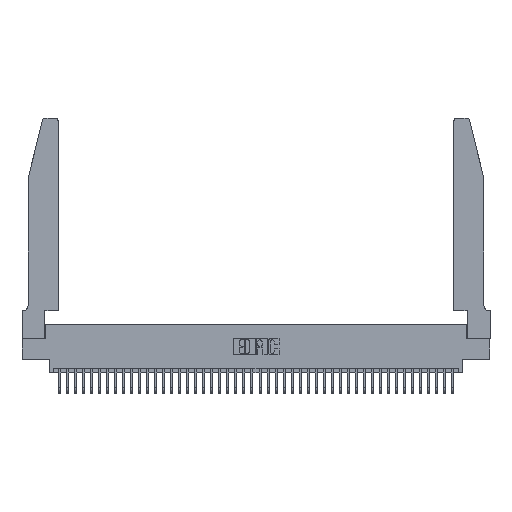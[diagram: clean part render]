
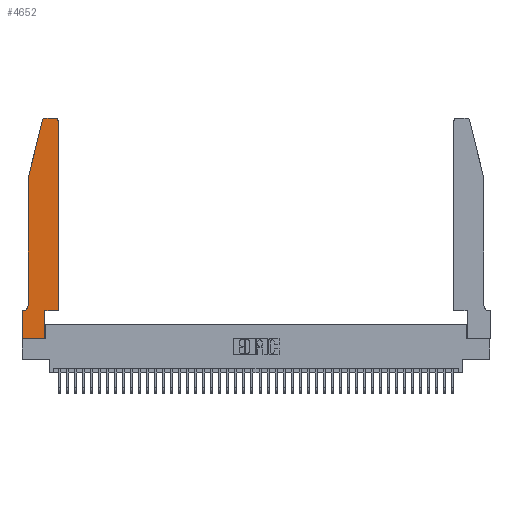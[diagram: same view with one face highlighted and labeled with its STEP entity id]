
A CAD part, top view. The second image highlights one B-rep face of the part: STEP entity #4652.
In plain terms, the highlighted planar face has unit normal (0, 0, 1).
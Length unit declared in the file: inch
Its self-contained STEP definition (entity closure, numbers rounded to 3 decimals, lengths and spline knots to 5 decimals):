
#1 = ORIENTED_EDGE ( 'NONE', *, *, #5140, .T. ) ;
#418 = CARTESIAN_POINT ( 'NONE',  ( 0.0755, 2., 0.37 ) ) ;
#725 = DIRECTION ( 'NONE',  ( -1., 0., 0. ) ) ;
#777 = EDGE_CURVE ( 'NONE', #25857, #13474, #34727, .T. ) ;
#866 = ORIENTED_EDGE ( 'NONE', *, *, #25130, .T. ) ;
#1638 = EDGE_CURVE ( 'NONE', #13474, #6282, #27188, .T. ) ;
#1708 = DIRECTION ( 'NONE',  ( 0., -1., 0. ) ) ;
#1858 = DIRECTION ( 'NONE',  ( 1., 0., 0. ) ) ;
#1869 = ORIENTED_EDGE ( 'NONE', *, *, #17423, .T. ) ;
#2972 = VERTEX_POINT ( 'NONE', #32875 ) ;
#3254 = CARTESIAN_POINT ( 'NONE',  ( 0.2605, 2.75, 0.37 ) ) ;
#3844 = DIRECTION ( 'NONE',  ( 0., 0., -1. ) ) ;
#4652 = ADVANCED_FACE ( 'NONE', ( #40376 ), #4885, .T. ) ;
#4885 = PLANE ( 'NONE',  #23230 ) ;
#5140 = EDGE_CURVE ( 'NONE', #6282, #18729, #25909, .T. ) ;
#6192 = DIRECTION ( 'NONE',  ( 0., 0., 1. ) ) ;
#6282 = VERTEX_POINT ( 'NONE', #31234 ) ;
#6352 = VECTOR ( 'NONE', #33932, 39.37008 ) ;
#7122 = CARTESIAN_POINT ( 'NONE',  ( 0.2865, 0.35, 0.37 ) ) ;
#7408 = LINE ( 'NONE', #8393, #6352 ) ;
#7755 = EDGE_LOOP ( 'NONE', ( #32621, #8436, #32282, #1, #1869, #41094, #28340, #11841, #17755, #16228, #40484, #866 ) ) ;
#8393 = CARTESIAN_POINT ( 'NONE',  ( 0.4505, 0.35, 0.37 ) ) ;
#8436 = ORIENTED_EDGE ( 'NONE', *, *, #777, .T. ) ;
#8941 = DIRECTION ( 'NONE',  ( 0., 1., 0. ) ) ;
#8959 = VERTEX_POINT ( 'NONE', #24991 ) ;
#9185 = VECTOR ( 'NONE', #19814, 39.37008 ) ;
#9940 = CIRCLE ( 'NONE', #27028, 0.03 ) ;
#11439 = DIRECTION ( 'NONE',  ( 1., 0., 0. ) ) ;
#11476 = CARTESIAN_POINT ( 'NONE',  ( 0.25487, 2.72718, 0.37 ) ) ;
#11786 = CARTESIAN_POINT ( 'NONE',  ( 0.2865, 0., 0.37 ) ) ;
#11841 = ORIENTED_EDGE ( 'NONE', *, *, #22970, .T. ) ;
#11880 = CARTESIAN_POINT ( 'NONE',  ( 0.284, 2.72, 0.37 ) ) ;
#11992 = LINE ( 'NONE', #30400, #27938 ) ;
#12754 = AXIS2_PLACEMENT_3D ( 'NONE', #11880, #34163, #15124 ) ;
#13474 = VERTEX_POINT ( 'NONE', #11476 ) ;
#14795 = CARTESIAN_POINT ( 'NONE',  ( 0.4505, 0.35, 0.37 ) ) ;
#15124 = DIRECTION ( 'NONE',  ( 1., 0., 0. ) ) ;
#16228 = ORIENTED_EDGE ( 'NONE', *, *, #28784, .T. ) ;
#17423 = EDGE_CURVE ( 'NONE', #18729, #35710, #30546, .T. ) ;
#17446 = VERTEX_POINT ( 'NONE', #7122 ) ;
#17754 = LINE ( 'NONE', #14795, #41091 ) ;
#17755 = ORIENTED_EDGE ( 'NONE', *, *, #26384, .T. ) ;
#18212 = CARTESIAN_POINT ( 'NONE',  ( 0.4505, 0.35, 0.37 ) ) ;
#18729 = VERTEX_POINT ( 'NONE', #28030 ) ;
#19696 = VERTEX_POINT ( 'NONE', #26534 ) ;
#19814 = DIRECTION ( 'NONE',  ( -0.239, -0.971, 0. ) ) ;
#21057 = CARTESIAN_POINT ( 'NONE',  ( 0.0755, 2., 0.37 ) ) ;
#21131 = CARTESIAN_POINT ( 'NONE',  ( 0., 0., 0.37 ) ) ;
#22970 = EDGE_CURVE ( 'NONE', #33814, #25055, #11992, .T. ) ;
#23080 = CARTESIAN_POINT ( 'NONE',  ( 0.0055, 0.42, 0.37 ) ) ;
#23230 = AXIS2_PLACEMENT_3D ( 'NONE', #27339, #30523, #11439 ) ;
#24111 = DIRECTION ( 'NONE',  ( 1., 0., 0. ) ) ;
#24272 = EDGE_CURVE ( 'NONE', #35710, #8959, #30805, .T. ) ;
#24288 = DIRECTION ( 'NONE',  ( 0., -1., 0. ) ) ;
#24928 = VECTOR ( 'NONE', #1708, 39.37008 ) ;
#24991 = CARTESIAN_POINT ( 'NONE',  ( 0., 0.35, 0.37 ) ) ;
#25027 = EDGE_CURVE ( 'NONE', #38772, #2972, #7408, .T. ) ;
#25055 = VERTEX_POINT ( 'NONE', #11786 ) ;
#25130 = EDGE_CURVE ( 'NONE', #2972, #19696, #9940, .T. ) ;
#25368 = CARTESIAN_POINT ( 'NONE',  ( 0.4205, 2.72, 0.37 ) ) ;
#25683 = DIRECTION ( 'NONE',  ( -1., 0., 0. ) ) ;
#25857 = VERTEX_POINT ( 'NONE', #28377 ) ;
#25909 = LINE ( 'NONE', #21057, #24928 ) ;
#26279 = DIRECTION ( 'NONE',  ( -1., 0., 0. ) ) ;
#26384 = EDGE_CURVE ( 'NONE', #25055, #17446, #33344, .T. ) ;
#26534 = CARTESIAN_POINT ( 'NONE',  ( 0.4205, 2.75, 0.37 ) ) ;
#27028 = AXIS2_PLACEMENT_3D ( 'NONE', #25368, #6192, #28616 ) ;
#27188 = LINE ( 'NONE', #418, #9185 ) ;
#27339 = CARTESIAN_POINT ( 'NONE',  ( 0., 0.35, 0.37 ) ) ;
#27938 = VECTOR ( 'NONE', #24111, 39.37008 ) ;
#28030 = CARTESIAN_POINT ( 'NONE',  ( 0.0755, 0.42, 0.37 ) ) ;
#28191 = EDGE_CURVE ( 'NONE', #8959, #33814, #31181, .T. ) ;
#28340 = ORIENTED_EDGE ( 'NONE', *, *, #28191, .T. ) ;
#28377 = CARTESIAN_POINT ( 'NONE',  ( 0.284, 2.75, 0.37 ) ) ;
#28616 = DIRECTION ( 'NONE',  ( 1., 0., 0. ) ) ;
#28784 = EDGE_CURVE ( 'NONE', #17446, #38772, #17754, .T. ) ;
#30400 = CARTESIAN_POINT ( 'NONE',  ( 0., 0., 0.37 ) ) ;
#30523 = DIRECTION ( 'NONE',  ( 0., 0., 1. ) ) ;
#30546 = CIRCLE ( 'NONE', #36730, 0.07 ) ;
#30805 = LINE ( 'NONE', #39133, #39297 ) ;
#31181 = LINE ( 'NONE', #21131, #38665 ) ;
#31234 = CARTESIAN_POINT ( 'NONE',  ( 0.0755, 2., 0.37 ) ) ;
#31263 = CARTESIAN_POINT ( 'NONE',  ( 0.2865, 0.35, 0.37 ) ) ;
#32114 = CARTESIAN_POINT ( 'NONE',  ( 0., 0., 0.37 ) ) ;
#32282 = ORIENTED_EDGE ( 'NONE', *, *, #1638, .T. ) ;
#32335 = VECTOR ( 'NONE', #8941, 39.37008 ) ;
#32621 = ORIENTED_EDGE ( 'NONE', *, *, #37240, .T. ) ;
#32875 = CARTESIAN_POINT ( 'NONE',  ( 0.4505, 2.72, 0.37 ) ) ;
#33240 = VECTOR ( 'NONE', #25683, 39.37008 ) ;
#33344 = LINE ( 'NONE', #31263, #32335 ) ;
#33814 = VERTEX_POINT ( 'NONE', #32114 ) ;
#33932 = DIRECTION ( 'NONE',  ( 0., 1., 0. ) ) ;
#34163 = DIRECTION ( 'NONE',  ( 0., 0., 1. ) ) ;
#34727 = CIRCLE ( 'NONE', #12754, 0.03 ) ;
#35710 = VERTEX_POINT ( 'NONE', #36719 ) ;
#36719 = CARTESIAN_POINT ( 'NONE',  ( 0.0055, 0.35, 0.37 ) ) ;
#36730 = AXIS2_PLACEMENT_3D ( 'NONE', #23080, #3844, #26279 ) ;
#37240 = EDGE_CURVE ( 'NONE', #19696, #25857, #39734, .T. ) ;
#38665 = VECTOR ( 'NONE', #24288, 39.37008 ) ;
#38772 = VERTEX_POINT ( 'NONE', #18212 ) ;
#39133 = CARTESIAN_POINT ( 'NONE',  ( 0.0755, 0.35, 0.37 ) ) ;
#39297 = VECTOR ( 'NONE', #725, 39.37008 ) ;
#39734 = LINE ( 'NONE', #3254, #33240 ) ;
#40376 = FACE_OUTER_BOUND ( 'NONE', #7755, .T. ) ;
#40484 = ORIENTED_EDGE ( 'NONE', *, *, #25027, .T. ) ;
#41091 = VECTOR ( 'NONE', #1858, 39.37008 ) ;
#41094 = ORIENTED_EDGE ( 'NONE', *, *, #24272, .T. ) ;
